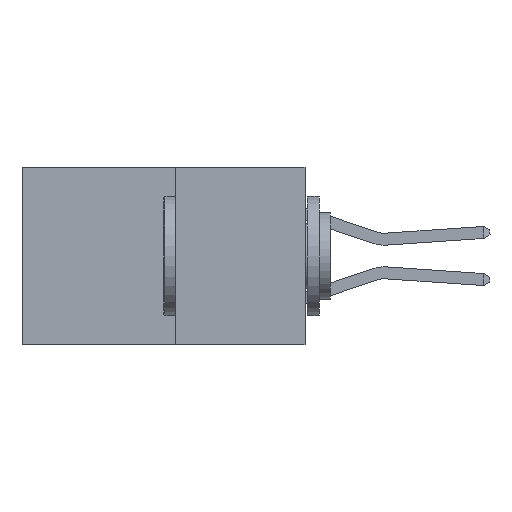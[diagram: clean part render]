
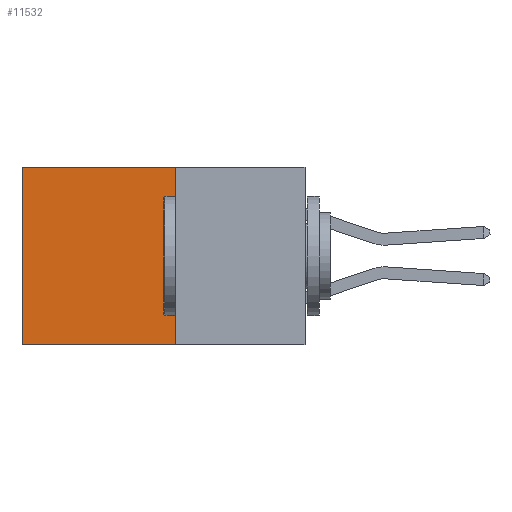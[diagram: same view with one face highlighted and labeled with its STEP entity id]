
A CAD part, left-side view. The second image highlights one B-rep face of the part: STEP entity #11532.
In plain terms, the highlighted planar face has unit normal (-1, 0, 0).
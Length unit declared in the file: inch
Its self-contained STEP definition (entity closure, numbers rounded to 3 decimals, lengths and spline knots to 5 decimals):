
#12 = LINE ( 'NONE', #12216, #13504 ) ;
#2116 = ORIENTED_EDGE ( 'NONE', *, *, #26168, .T. ) ;
#3016 = VERTEX_POINT ( 'NONE', #24459 ) ;
#3225 = VECTOR ( 'NONE', #23366, 39.37008 ) ;
#3395 = CARTESIAN_POINT ( 'NONE',  ( 0.277, 0.27, -0.37 ) ) ;
#3469 = ORIENTED_EDGE ( 'NONE', *, *, #21258, .F. ) ;
#4302 = ORIENTED_EDGE ( 'NONE', *, *, #23686, .F. ) ;
#4700 = PLANE ( 'NONE',  #8456 ) ;
#7421 = DIRECTION ( 'NONE',  ( 0., 0., -1. ) ) ;
#7913 = FACE_OUTER_BOUND ( 'NONE', #21334, .T. ) ;
#8456 = AXIS2_PLACEMENT_3D ( 'NONE', #18041, #23289, #7421 ) ;
#10119 = CARTESIAN_POINT ( 'NONE',  ( 0.277, 0.59, -0.37 ) ) ;
#10168 = CARTESIAN_POINT ( 'NONE',  ( 0.277, 0.59, 0. ) ) ;
#11532 = ADVANCED_FACE ( 'NONE', ( #7913 ), #4700, .F. ) ;
#11714 = VECTOR ( 'NONE', #24644, 39.37008 ) ;
#12216 = CARTESIAN_POINT ( 'NONE',  ( 0.277, 0.27, 0. ) ) ;
#12542 = LINE ( 'NONE', #3395, #11714 ) ;
#13504 = VECTOR ( 'NONE', #25405, 39.37008 ) ;
#13598 = LINE ( 'NONE', #28902, #26752 ) ;
#16200 = VERTEX_POINT ( 'NONE', #26022 ) ;
#17835 = EDGE_CURVE ( 'NONE', #20918, #3016, #24427, .T. ) ;
#18041 = CARTESIAN_POINT ( 'NONE',  ( 0.277, 0.27, -0.37 ) ) ;
#19092 = CARTESIAN_POINT ( 'NONE',  ( 0.277, 0.27, -0.37 ) ) ;
#20918 = VERTEX_POINT ( 'NONE', #10168 ) ;
#21258 = EDGE_CURVE ( 'NONE', #29270, #3016, #12542, .T. ) ;
#21334 = EDGE_LOOP ( 'NONE', ( #33369, #3469, #4302, #2116 ) ) ;
#23289 = DIRECTION ( 'NONE',  ( 1., 0., 0. ) ) ;
#23366 = DIRECTION ( 'NONE',  ( 0., 0., -1. ) ) ;
#23686 = EDGE_CURVE ( 'NONE', #16200, #29270, #13598, .T. ) ;
#24427 = LINE ( 'NONE', #10119, #3225 ) ;
#24459 = CARTESIAN_POINT ( 'NONE',  ( 0.277, 0.59, -0.37 ) ) ;
#24644 = DIRECTION ( 'NONE',  ( 0., 1., 0. ) ) ;
#25405 = DIRECTION ( 'NONE',  ( 0., 1., 0. ) ) ;
#26022 = CARTESIAN_POINT ( 'NONE',  ( 0.277, 0.27, 0. ) ) ;
#26168 = EDGE_CURVE ( 'NONE', #16200, #20918, #12, .T. ) ;
#26752 = VECTOR ( 'NONE', #31500, 39.37008 ) ;
#28902 = CARTESIAN_POINT ( 'NONE',  ( 0.277, 0.27, -0.37 ) ) ;
#29270 = VERTEX_POINT ( 'NONE', #19092 ) ;
#31500 = DIRECTION ( 'NONE',  ( 0., 0., -1. ) ) ;
#33369 = ORIENTED_EDGE ( 'NONE', *, *, #17835, .T. ) ;
